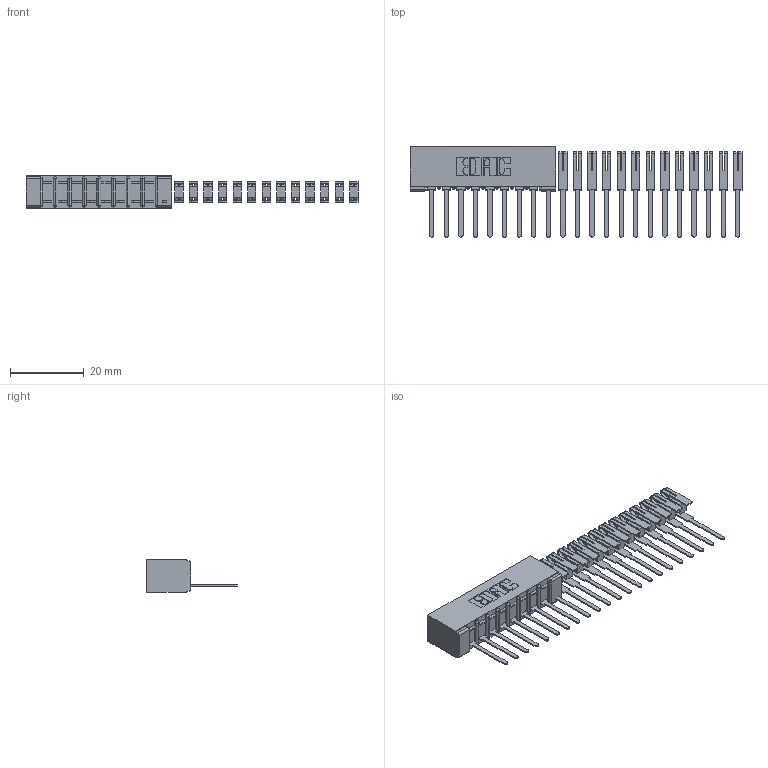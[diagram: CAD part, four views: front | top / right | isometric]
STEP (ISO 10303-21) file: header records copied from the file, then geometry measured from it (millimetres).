
FILE_DESCRIPTION (( 'STEP AP203' ), '1' );
FILE_NAME ('357-022-541-101.STEP', '2018-08-08T22:18:22', ( '' ), ( '' ), 'SwSTEP 2.0', 'SolidWorks 2016', '' );
FILE_SCHEMA (( 'CONFIG_CONTROL_DESIGN' ));
Length unit declared in the file: inch
Products named in the file (3): 307 Part_No Mounting Lugs; 307-290-002_541; 357-022-541-101
Assembly tree (23 placements, depth 2):
  357-022-541-101
    307 Part_No Mounting Lugs
    307-290-002_541  x22
Bounding box: 90.26 x 24.59 x 8.71 mm (x, y, z)
Volume: 3314.7 mm3; surface area: 8493.5 mm2
Topology: 23 solids, 23 shells, 1467 faces, 4507 edges, 2978 vertices
Faces by surface type: plane 888, cylinder 561, sphere 18
Entity records: 11938 total; most frequent: CARTESIAN_POINT 1946, ORIENTED_EDGE 1922, DIRECTION 1919, EDGE_CURVE 961, VECTOR 721, LINE 721, VERTEX_POINT 626, AXIS2_PLACEMENT_3D 599
